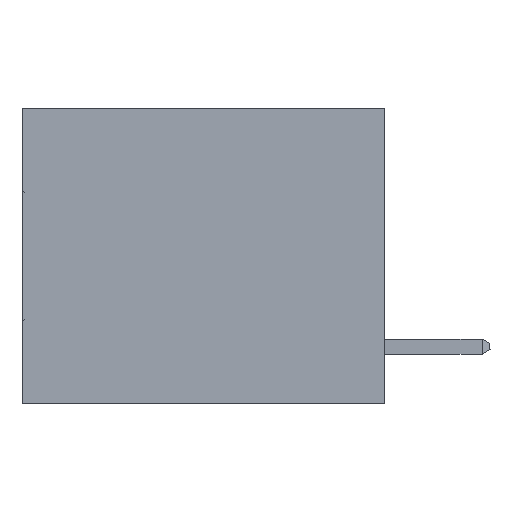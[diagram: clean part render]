
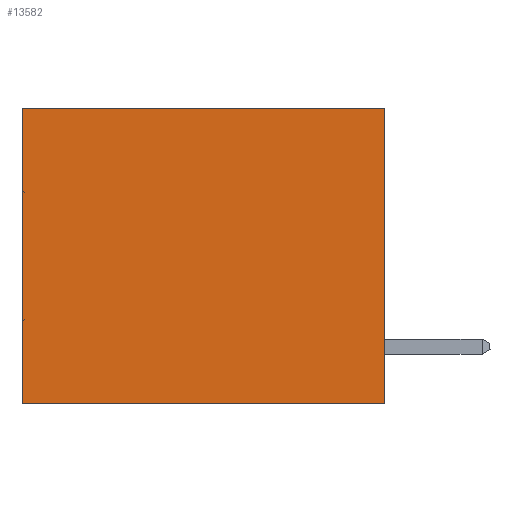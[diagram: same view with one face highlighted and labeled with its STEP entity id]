
A CAD part, left-side view. The second image highlights one B-rep face of the part: STEP entity #13582.
In plain terms, the highlighted planar face has unit normal (-1, 0, 0).
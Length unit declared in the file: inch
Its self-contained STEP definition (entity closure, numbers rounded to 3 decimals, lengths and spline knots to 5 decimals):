
#2465 = CARTESIAN_POINT ( 'NONE',  ( 0.3165, 0., 0. ) ) ;
#3319 = EDGE_CURVE ( 'NONE', #32403, #15154, #16065, .T. ) ;
#5471 = ORIENTED_EDGE ( 'NONE', *, *, #17058, .T. ) ;
#5646 = CARTESIAN_POINT ( 'NONE',  ( 0.3165, 0., -0.49 ) ) ;
#6552 = LINE ( 'NONE', #13507, #27193 ) ;
#7325 = EDGE_CURVE ( 'NONE', #8229, #32403, #33949, .T. ) ;
#8229 = VERTEX_POINT ( 'NONE', #2465 ) ;
#8818 = CARTESIAN_POINT ( 'NONE',  ( 0.3165, 0.6, -0.49 ) ) ;
#9592 = VECTOR ( 'NONE', #10679, 39.37008 ) ;
#9790 = ORIENTED_EDGE ( 'NONE', *, *, #3319, .F. ) ;
#10679 = DIRECTION ( 'NONE',  ( 0., 0., -1. ) ) ;
#10698 = EDGE_CURVE ( 'NONE', #13366, #15154, #25146, .T. ) ;
#10783 = ORIENTED_EDGE ( 'NONE', *, *, #10698, .T. ) ;
#10845 = DIRECTION ( 'NONE',  ( 0., 1., 0. ) ) ;
#11394 = ORIENTED_EDGE ( 'NONE', *, *, #7325, .F. ) ;
#11825 = DIRECTION ( 'NONE',  ( 1., 0., 0. ) ) ;
#13366 = VERTEX_POINT ( 'NONE', #26729 ) ;
#13507 = CARTESIAN_POINT ( 'NONE',  ( 0.3165, 0., 0. ) ) ;
#13582 = ADVANCED_FACE ( 'NONE', ( #26941 ), #30177, .F. ) ;
#14330 = DIRECTION ( 'NONE',  ( 0., 0., -1. ) ) ;
#15154 = VERTEX_POINT ( 'NONE', #8818 ) ;
#16065 = LINE ( 'NONE', #24146, #20267 ) ;
#16404 = VECTOR ( 'NONE', #33925, 39.37008 ) ;
#16765 = CARTESIAN_POINT ( 'NONE',  ( 0.3165, 0.6, -0.49 ) ) ;
#17009 = CARTESIAN_POINT ( 'NONE',  ( 0.3165, 0., -0.49 ) ) ;
#17058 = EDGE_CURVE ( 'NONE', #8229, #13366, #6552, .T. ) ;
#20267 = VECTOR ( 'NONE', #29229, 39.37008 ) ;
#24146 = CARTESIAN_POINT ( 'NONE',  ( 0.3165, 0., -0.49 ) ) ;
#25146 = LINE ( 'NONE', #16765, #16404 ) ;
#25949 = EDGE_LOOP ( 'NONE', ( #10783, #9790, #11394, #5471 ) ) ;
#26729 = CARTESIAN_POINT ( 'NONE',  ( 0.3165, 0.6, 0. ) ) ;
#26941 = FACE_OUTER_BOUND ( 'NONE', #25949, .T. ) ;
#27193 = VECTOR ( 'NONE', #10845, 39.37008 ) ;
#27737 = AXIS2_PLACEMENT_3D ( 'NONE', #17009, #11825, #14330 ) ;
#29023 = CARTESIAN_POINT ( 'NONE',  ( 0.3165, 0., -0.49 ) ) ;
#29229 = DIRECTION ( 'NONE',  ( 0., 1., 0. ) ) ;
#30177 = PLANE ( 'NONE',  #27737 ) ;
#32403 = VERTEX_POINT ( 'NONE', #29023 ) ;
#33925 = DIRECTION ( 'NONE',  ( 0., 0., -1. ) ) ;
#33949 = LINE ( 'NONE', #5646, #9592 ) ;
